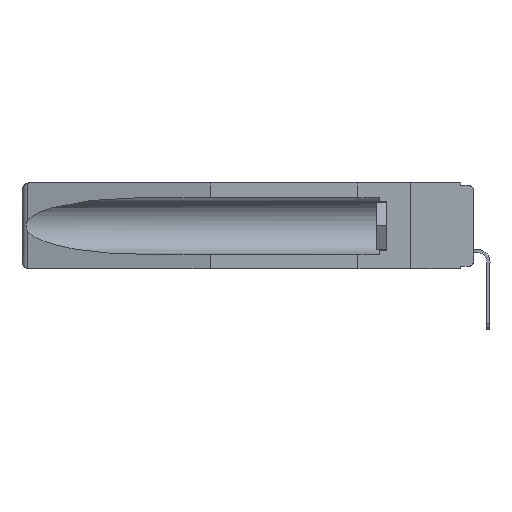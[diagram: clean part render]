
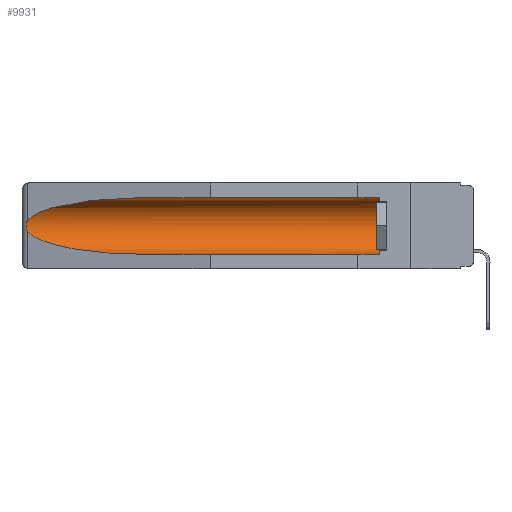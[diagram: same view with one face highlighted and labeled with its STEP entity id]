
A CAD part, left-side view. The second image highlights one B-rep face of the part: STEP entity #9931.
In plain terms, the highlighted cylindrical face has radius 2.857 mm (diameter 5.715 mm), a partial arc.
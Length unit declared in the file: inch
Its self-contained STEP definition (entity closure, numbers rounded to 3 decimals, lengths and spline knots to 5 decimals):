
#89 = VECTOR ( 'NONE', #3177, 39.37008 ) ;
#151 = DIRECTION ( 'NONE',  ( 0., 0., 1. ) ) ;
#671 = EDGE_CURVE ( 'NONE', #14168, #7635, #13497, .T. ) ;
#908 = ORIENTED_EDGE ( 'NONE', *, *, #671, .T. ) ;
#1110 = FACE_OUTER_BOUND ( 'NONE', #12253, .T. ) ;
#1131 = DIRECTION ( 'NONE',  ( 0., 1., 0. ) ) ;
#2086 = CARTESIAN_POINT ( 'NONE',  ( 0.155, 1.07973, -0.284 ) ) ;
#2099 = EDGE_CURVE ( 'NONE', #7635, #6626, #9022, .T. ) ;
#2167 = LINE ( 'NONE', #11797, #8222 ) ;
#2393 = CARTESIAN_POINT ( 'NONE',  ( 0.21114, 1.30732, -0.059 ) ) ;
#3029 = EDGE_CURVE ( 'NONE', #15357, #14168, #4187, .T. ) ;
#3108 = CARTESIAN_POINT ( 'NONE',  ( 0.155, 0.126, -0.284 ) ) ;
#3177 = DIRECTION ( 'NONE',  ( 0., 1., 0. ) ) ;
#3548 = CARTESIAN_POINT ( 'NONE',  ( 0.26537, 1.52718, -0.14972 ) ) ;
#3554 = CARTESIAN_POINT ( 'NONE',  ( 0.26537, 1.52718, -0.14972 ) ) ;
#3692 = AXIS2_PLACEMENT_3D ( 'NONE', #4817, #11067, #151 ) ;
#4001 = CARTESIAN_POINT ( 'NONE',  ( 0.26537, 1.52718, -0.19328 ) ) ;
#4088 = CARTESIAN_POINT ( 'NONE',  ( 0.26597, 1.5296, -0.19026 ) ) ;
#4187 =( BOUNDED_CURVE ( )  B_SPLINE_CURVE ( 3, ( #10832, #2393, #4721, #14504 ),
 .UNSPECIFIED., .F., .F. ) 
 B_SPLINE_CURVE_WITH_KNOTS ( ( 4, 4 ),
 ( 4.71239, 6.08839 ),
 .UNSPECIFIED. ) 
 CURVE ( )  GEOMETRIC_REPRESENTATION_ITEM ( )  RATIONAL_B_SPLINE_CURVE ( ( 1., 0.848, 0.848, 1. ) ) 
 REPRESENTATION_ITEM ( '' )  );
#4334 = ORIENTED_EDGE ( 'NONE', *, *, #3029, .T. ) ;
#4721 = CARTESIAN_POINT ( 'NONE',  ( 0.25451, 1.48313, -0.09465 ) ) ;
#4777 = CARTESIAN_POINT ( 'NONE',  ( 0.155, 1.07973, -0.284 ) ) ;
#4817 = CARTESIAN_POINT ( 'NONE',  ( 0.155, 0.126, -0.1715 ) ) ;
#4842 = CARTESIAN_POINT ( 'NONE',  ( 0.26654, 1.53092, -0.15636 ) ) ;
#5212 = VERTEX_POINT ( 'NONE', #3108 ) ;
#5238 = CARTESIAN_POINT ( 'NONE',  ( 0.2675, 1.53308, -0.16763 ) ) ;
#5404 = CARTESIAN_POINT ( 'NONE',  ( 0.26537, 1.52718, -0.19328 ) ) ;
#6012 = CYLINDRICAL_SURFACE ( 'NONE', #7495, 0.1125 ) ;
#6579 = EDGE_CURVE ( 'NONE', #5212, #6626, #2167, .T. ) ;
#6626 = VERTEX_POINT ( 'NONE', #2086 ) ;
#6742 = ORIENTED_EDGE ( 'NONE', *, *, #12522, .T. ) ;
#7319 = CIRCLE ( 'NONE', #3692, 0.1125 ) ;
#7495 = AXIS2_PLACEMENT_3D ( 'NONE', #9772, #15751, #14571 ) ;
#7635 = VERTEX_POINT ( 'NONE', #4001 ) ;
#7895 = CARTESIAN_POINT ( 'NONE',  ( 0.2673, 1.53269, -0.17917 ) ) ;
#7940 = LINE ( 'NONE', #11614, #89 ) ;
#8222 = VECTOR ( 'NONE', #1131, 39.37008 ) ;
#9022 =( BOUNDED_CURVE ( )  B_SPLINE_CURVE ( 3, ( #14482, #13287, #14248, #4777 ),
 .UNSPECIFIED., .F., .F. ) 
 B_SPLINE_CURVE_WITH_KNOTS ( ( 4, 4 ),
 ( 0.1948, 1.5708 ),
 .UNSPECIFIED. ) 
 CURVE ( )  GEOMETRIC_REPRESENTATION_ITEM ( )  RATIONAL_B_SPLINE_CURVE ( ( 1., 0.848, 0.848, 1. ) ) 
 REPRESENTATION_ITEM ( '' )  );
#9609 = ORIENTED_EDGE ( 'NONE', *, *, #9738, .T. ) ;
#9738 = EDGE_CURVE ( 'NONE', #12954, #15357, #7940, .T. ) ;
#9747 = CARTESIAN_POINT ( 'NONE',  ( 0.2673, 1.5327, -0.16383 ) ) ;
#9772 = CARTESIAN_POINT ( 'NONE',  ( 0.155, -0.30754, -0.1715 ) ) ;
#9931 = ADVANCED_FACE ( 'NONE', ( #1110 ), #6012, .F. ) ;
#10832 = CARTESIAN_POINT ( 'NONE',  ( 0.155, 1.07973, -0.059 ) ) ;
#10947 = CARTESIAN_POINT ( 'NONE',  ( 0.26597, 1.52961, -0.15275 ) ) ;
#11067 = DIRECTION ( 'NONE',  ( 0., -1., 0. ) ) ;
#11328 = CARTESIAN_POINT ( 'NONE',  ( 0.26655, 1.53094, -0.18657 ) ) ;
#11510 = CARTESIAN_POINT ( 'NONE',  ( 0.155, 1.07973, -0.059 ) ) ;
#11614 = CARTESIAN_POINT ( 'NONE',  ( 0.155, -0.30754, -0.059 ) ) ;
#11797 = CARTESIAN_POINT ( 'NONE',  ( 0.155, -0.30754, -0.284 ) ) ;
#12253 = EDGE_LOOP ( 'NONE', ( #4334, #908, #14225, #14399, #6742, #9609 ) ) ;
#12522 = EDGE_CURVE ( 'NONE', #5212, #12954, #7319, .T. ) ;
#12612 = CARTESIAN_POINT ( 'NONE',  ( 0.2675, 1.53308, -0.17534 ) ) ;
#12954 = VERTEX_POINT ( 'NONE', #14342 ) ;
#13287 = CARTESIAN_POINT ( 'NONE',  ( 0.25451, 1.48313, -0.24835 ) ) ;
#13497 = B_SPLINE_CURVE_WITH_KNOTS ( 'NONE', 3,
 ( #3548, #10947, #4842, #9747, #5238, #12612, #7895, #11328, #4088, #5404 ),
 .UNSPECIFIED., .F., .F.,
 ( 4, 2, 2, 2, 4 ),
 ( 0., 0.00029, 0.00058, 0.00087, 0.00117 ),
 .UNSPECIFIED. ) ;
#14168 = VERTEX_POINT ( 'NONE', #3554 ) ;
#14225 = ORIENTED_EDGE ( 'NONE', *, *, #2099, .T. ) ;
#14248 = CARTESIAN_POINT ( 'NONE',  ( 0.21114, 1.30732, -0.284 ) ) ;
#14342 = CARTESIAN_POINT ( 'NONE',  ( 0.155, 0.126, -0.059 ) ) ;
#14399 = ORIENTED_EDGE ( 'NONE', *, *, #6579, .F. ) ;
#14482 = CARTESIAN_POINT ( 'NONE',  ( 0.26537, 1.52718, -0.19328 ) ) ;
#14504 = CARTESIAN_POINT ( 'NONE',  ( 0.26537, 1.52718, -0.14972 ) ) ;
#14571 = DIRECTION ( 'NONE',  ( 0., 0., 1. ) ) ;
#15357 = VERTEX_POINT ( 'NONE', #11510 ) ;
#15751 = DIRECTION ( 'NONE',  ( 0., 1., 0. ) ) ;
